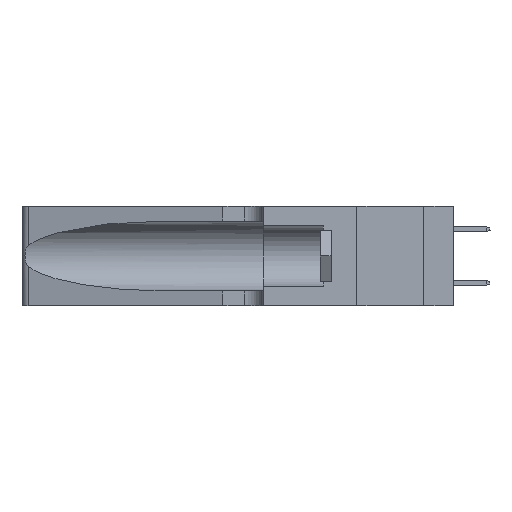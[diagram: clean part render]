
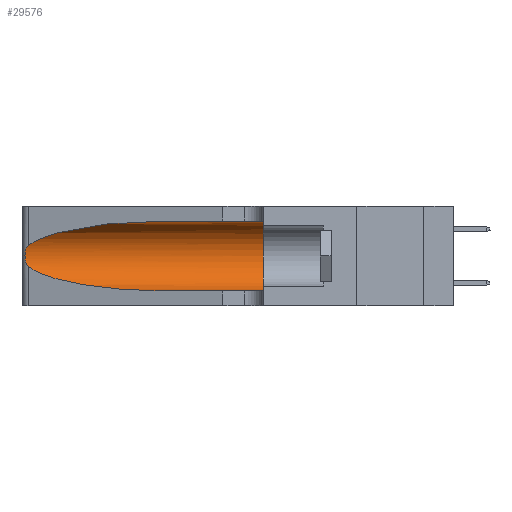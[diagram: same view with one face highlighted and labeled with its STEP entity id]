
A CAD part, left-side view. The second image highlights one B-rep face of the part: STEP entity #29576.
In plain terms, the highlighted cylindrical face has radius 3.308 mm (diameter 6.617 mm), a partial arc.
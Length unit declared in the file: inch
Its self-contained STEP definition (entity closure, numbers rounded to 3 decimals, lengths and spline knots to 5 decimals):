
#125 = LINE ( 'NONE', #12213, #331 ) ;
#331 = VECTOR ( 'NONE', #2572, 39.37008 ) ;
#549 = CARTESIAN_POINT ( 'NONE',  ( 0.1305, 0.72297, 0.31525 ) ) ;
#876 = VERTEX_POINT ( 'NONE', #549 ) ;
#929 = CIRCLE ( 'NONE', #22563, 0.13025 ) ;
#2169 = EDGE_CURVE ( 'NONE', #5524, #11353, #125, .T. ) ;
#2572 = DIRECTION ( 'NONE',  ( 0., -1., 0. ) ) ;
#2740 = CARTESIAN_POINT ( 'NONE',  ( 0.1305, 0.35, 0.05475 ) ) ;
#3156 = VECTOR ( 'NONE', #17889, 39.37008 ) ;
#5524 = VERTEX_POINT ( 'NONE', #11280 ) ;
#5705 = CARTESIAN_POINT ( 'NONE',  ( 0.26075, 1.23896, 0.178 ) ) ;
#5958 = ORIENTED_EDGE ( 'NONE', *, *, #29051, .F. ) ;
#6292 =( BOUNDED_CURVE ( )  B_SPLINE_CURVE ( 3, ( #14570, #39411, #7578, #27111 ),
 .UNSPECIFIED., .F., .F. ) 
 B_SPLINE_CURVE_WITH_KNOTS ( ( 4, 4 ),
 ( 1.5708, 2.84003 ),
 .UNSPECIFIED. ) 
 CURVE ( )  GEOMETRIC_REPRESENTATION_ITEM ( )  RATIONAL_B_SPLINE_CURVE ( ( 1., 0.87, 0.87, 1. ) ) 
 REPRESENTATION_ITEM ( '' )  );
#6319 = CARTESIAN_POINT ( 'NONE',  ( 0.1305, 1.61858, 0.185 ) ) ;
#7169 = EDGE_CURVE ( 'NONE', #26664, #5524, #35699, .T. ) ;
#7578 = CARTESIAN_POINT ( 'NONE',  ( 0.2373, 1.15595, 0.28018 ) ) ;
#8597 = CARTESIAN_POINT ( 'NONE',  ( 0.25487, 1.22718, 0.22369 ) ) ;
#8916 = CARTESIAN_POINT ( 'NONE',  ( 0.18966, 0.96281, 0.05475 ) ) ;
#9425 = CARTESIAN_POINT ( 'NONE',  ( 0.25555, 1.22993, 0.14849 ) ) ;
#9429 = CYLINDRICAL_SURFACE ( 'NONE', #11058, 0.13025 ) ;
#10720 = CARTESIAN_POINT ( 'NONE',  ( 0.25487, 1.22718, 0.22369 ) ) ;
#11058 = AXIS2_PLACEMENT_3D ( 'NONE', #6319, #18251, #33877 ) ;
#11280 = CARTESIAN_POINT ( 'NONE',  ( 0.1305, 0.72297, 0.05475 ) ) ;
#11353 = VERTEX_POINT ( 'NONE', #2740 ) ;
#12084 = CARTESIAN_POINT ( 'NONE',  ( 0.25787, 1.23484, 0.2124 ) ) ;
#12213 = CARTESIAN_POINT ( 'NONE',  ( 0.1305, 1.61858, 0.05475 ) ) ;
#13450 = EDGE_CURVE ( 'NONE', #29797, #11353, #929, .T. ) ;
#13627 = ORIENTED_EDGE ( 'NONE', *, *, #19997, .T. ) ;
#14570 = CARTESIAN_POINT ( 'NONE',  ( 0.1305, 0.72297, 0.31525 ) ) ;
#14978 = CARTESIAN_POINT ( 'NONE',  ( 0.25487, 1.22718, 0.14631 ) ) ;
#15180 = CARTESIAN_POINT ( 'NONE',  ( 0.25789, 1.23486, 0.15765 ) ) ;
#15386 = CARTESIAN_POINT ( 'NONE',  ( 0.25856, 1.23593, 0.16098 ) ) ;
#17537 = DIRECTION ( 'NONE',  ( 0., 1., 0. ) ) ;
#17889 = DIRECTION ( 'NONE',  ( 0., -1., 0. ) ) ;
#18192 = EDGE_LOOP ( 'NONE', ( #13627, #19773, #25618, #39456, #35283, #5958 ) ) ;
#18251 = DIRECTION ( 'NONE',  ( 0., -1., 0. ) ) ;
#18654 = CARTESIAN_POINT ( 'NONE',  ( 0.25854, 1.2359, 0.20912 ) ) ;
#19773 = ORIENTED_EDGE ( 'NONE', *, *, #20151, .T. ) ;
#19997 = EDGE_CURVE ( 'NONE', #876, #28799, #6292, .T. ) ;
#20151 = EDGE_CURVE ( 'NONE', #28799, #26664, #26318, .T. ) ;
#20837 = DIRECTION ( 'NONE',  ( 0., 0., 1. ) ) ;
#21348 = FACE_OUTER_BOUND ( 'NONE', #18192, .T. ) ;
#21736 = CARTESIAN_POINT ( 'NONE',  ( 0.25639, 1.23184, 0.21858 ) ) ;
#21911 = CARTESIAN_POINT ( 'NONE',  ( 0.25487, 1.22718, 0.14631 ) ) ;
#21938 = CARTESIAN_POINT ( 'NONE',  ( 0.25639, 1.23186, 0.15144 ) ) ;
#22255 = CARTESIAN_POINT ( 'NONE',  ( 0.1305, 0.72297, 0.05475 ) ) ;
#22563 = AXIS2_PLACEMENT_3D ( 'NONE', #33163, #17537, #20837 ) ;
#23879 = LINE ( 'NONE', #36372, #3156 ) ;
#25058 = CARTESIAN_POINT ( 'NONE',  ( 0.26075, 1.23896, 0.19203 ) ) ;
#25618 = ORIENTED_EDGE ( 'NONE', *, *, #7169, .T. ) ;
#26318 = B_SPLINE_CURVE_WITH_KNOTS ( 'NONE', 3,
 ( #8597, #30793, #21736, #12084, #18654, #33875, #25058, #5705, #37551, #15386, #15180, #21938, #9425, #14978 ),
 .UNSPECIFIED., .F., .F.,
 ( 4, 2, 2, 2, 2, 2, 4 ),
 ( 0., 0.00027, 0.00053, 0.00107, 0.0016, 0.00187, 0.00214 ),
 .UNSPECIFIED. ) ;
#26664 = VERTEX_POINT ( 'NONE', #21911 ) ;
#27111 = CARTESIAN_POINT ( 'NONE',  ( 0.25487, 1.22718, 0.22369 ) ) ;
#28799 = VERTEX_POINT ( 'NONE', #10720 ) ;
#29051 = EDGE_CURVE ( 'NONE', #876, #29797, #23879, .T. ) ;
#29576 = ADVANCED_FACE ( 'NONE', ( #21348 ), #9429, .F. ) ;
#29797 = VERTEX_POINT ( 'NONE', #37751 ) ;
#30793 = CARTESIAN_POINT ( 'NONE',  ( 0.25555, 1.22994, 0.2215 ) ) ;
#31108 = CARTESIAN_POINT ( 'NONE',  ( 0.25487, 1.22718, 0.14631 ) ) ;
#33163 = CARTESIAN_POINT ( 'NONE',  ( 0.1305, 0.35, 0.185 ) ) ;
#33875 = CARTESIAN_POINT ( 'NONE',  ( 0.26018, 1.23835, 0.19895 ) ) ;
#33877 = DIRECTION ( 'NONE',  ( 0., 0., -1. ) ) ;
#35283 = ORIENTED_EDGE ( 'NONE', *, *, #13450, .F. ) ;
#35699 =( BOUNDED_CURVE ( )  B_SPLINE_CURVE ( 3, ( #31108, #37849, #8916, #22255 ),
 .UNSPECIFIED., .F., .F. ) 
 B_SPLINE_CURVE_WITH_KNOTS ( ( 4, 4 ),
 ( 3.44316, 4.71239 ),
 .UNSPECIFIED. ) 
 CURVE ( )  GEOMETRIC_REPRESENTATION_ITEM ( )  RATIONAL_B_SPLINE_CURVE ( ( 1., 0.87, 0.87, 1. ) ) 
 REPRESENTATION_ITEM ( '' )  );
#36372 = CARTESIAN_POINT ( 'NONE',  ( 0.1305, 1.61858, 0.31525 ) ) ;
#37551 = CARTESIAN_POINT ( 'NONE',  ( 0.26017, 1.23833, 0.17102 ) ) ;
#37751 = CARTESIAN_POINT ( 'NONE',  ( 0.1305, 0.35, 0.31525 ) ) ;
#37849 = CARTESIAN_POINT ( 'NONE',  ( 0.2373, 1.15595, 0.08982 ) ) ;
#39411 = CARTESIAN_POINT ( 'NONE',  ( 0.18966, 0.96281, 0.31525 ) ) ;
#39456 = ORIENTED_EDGE ( 'NONE', *, *, #2169, .T. ) ;
